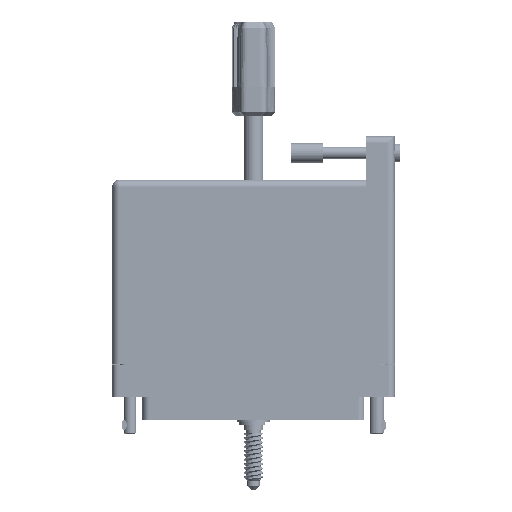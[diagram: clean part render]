
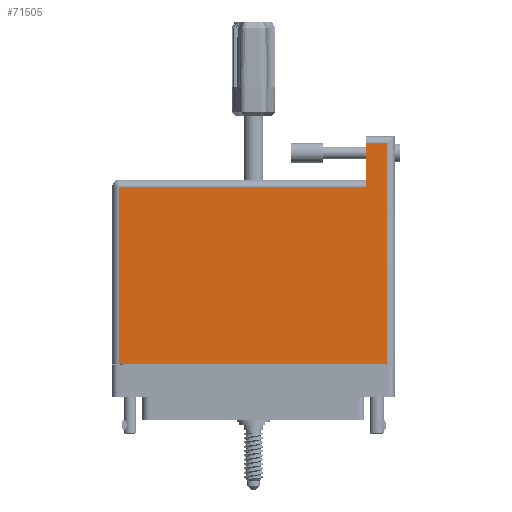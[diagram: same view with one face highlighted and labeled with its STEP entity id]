
A CAD part, front view. The second image highlights one B-rep face of the part: STEP entity #71505.
In plain terms, the highlighted face is planar.
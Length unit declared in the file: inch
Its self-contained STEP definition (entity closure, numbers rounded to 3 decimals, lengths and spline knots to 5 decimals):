
#1903 = ORIENTED_EDGE ( 'NONE', *, *, #75882, .T. ) ;
#1922 = VERTEX_POINT ( 'NONE', #93160 ) ;
#2564 = VERTEX_POINT ( 'NONE', #86191 ) ;
#4889 = VECTOR ( 'NONE', #37113, 39.37008 ) ;
#7090 = VECTOR ( 'NONE', #66469, 39.37008 ) ;
#7137 = CARTESIAN_POINT ( 'NONE',  ( 1.289, -0.1, 0.617 ) ) ;
#7687 = LINE ( 'NONE', #44389, #44986 ) ;
#10917 = EDGE_CURVE ( 'NONE', #56091, #29595, #30748, .T. ) ;
#13269 = ORIENTED_EDGE ( 'NONE', *, *, #47690, .T. ) ;
#14155 = AXIS2_PLACEMENT_3D ( 'NONE', #52039, #90207, #36883 ) ;
#15061 = CARTESIAN_POINT ( 'NONE',  ( -1.359, 2.025, 0.617 ) ) ;
#16395 = LINE ( 'NONE', #59484, #85983 ) ;
#24014 = DIRECTION ( 'NONE',  ( 0., -1., 0. ) ) ;
#25259 = ORIENTED_EDGE ( 'NONE', *, *, #70990, .T. ) ;
#27114 = DIRECTION ( 'NONE',  ( 1., 0., 0. ) ) ;
#29595 = VERTEX_POINT ( 'NONE', #50216 ) ;
#30748 = LINE ( 'NONE', #73796, #7090 ) ;
#36883 = DIRECTION ( 'NONE',  ( -1., 0., 0. ) ) ;
#37003 = DIRECTION ( 'NONE',  ( 0., -1., 0. ) ) ;
#37113 = DIRECTION ( 'NONE',  ( -1., 0., 0. ) ) ;
#41360 = CARTESIAN_POINT ( 'NONE',  ( -1.289, -0.1, 0.617 ) ) ;
#44389 = CARTESIAN_POINT ( 'NONE',  ( 1.289, 2.095, 0.617 ) ) ;
#44986 = VECTOR ( 'NONE', #67366, 39.37008 ) ;
#45047 = CARTESIAN_POINT ( 'NONE',  ( -1.289, -0.1, 0.617 ) ) ;
#47378 = VECTOR ( 'NONE', #27114, 39.37008 ) ;
#47690 = EDGE_CURVE ( 'NONE', #53337, #94446, #69347, .T. ) ;
#50216 = CARTESIAN_POINT ( 'NONE',  ( -1.289, 1.605, 0.617 ) ) ;
#52039 = CARTESIAN_POINT ( 'NONE',  ( -1.359, 1.675, 0.617 ) ) ;
#53337 = VERTEX_POINT ( 'NONE', #41360 ) ;
#55334 = EDGE_CURVE ( 'NONE', #94446, #1922, #7687, .T. ) ;
#55707 = EDGE_LOOP ( 'NONE', ( #65837, #84971, #13269, #86578, #1903, #25259 ) ) ;
#56091 = VERTEX_POINT ( 'NONE', #71416 ) ;
#59484 = CARTESIAN_POINT ( 'NONE',  ( 1.079, 2.095, 0.617 ) ) ;
#61032 = LINE ( 'NONE', #15061, #4889 ) ;
#65837 = ORIENTED_EDGE ( 'NONE', *, *, #10917, .T. ) ;
#66469 = DIRECTION ( 'NONE',  ( -1., 0., 0. ) ) ;
#67366 = DIRECTION ( 'NONE',  ( 0., 1., 0. ) ) ;
#67667 = PLANE ( 'NONE',  #14155 ) ;
#69347 = LINE ( 'NONE', #91891, #47378 ) ;
#70990 = EDGE_CURVE ( 'NONE', #2564, #56091, #16395, .T. ) ;
#71416 = CARTESIAN_POINT ( 'NONE',  ( 1.079, 1.605, 0.617 ) ) ;
#71505 = ADVANCED_FACE ( 'NONE', ( #90671 ), #67667, .F. ) ;
#73796 = CARTESIAN_POINT ( 'NONE',  ( -1.359, 1.605, 0.617 ) ) ;
#75882 = EDGE_CURVE ( 'NONE', #1922, #2564, #61032, .T. ) ;
#84971 = ORIENTED_EDGE ( 'NONE', *, *, #85835, .T. ) ;
#85835 = EDGE_CURVE ( 'NONE', #29595, #53337, #91032, .T. ) ;
#85983 = VECTOR ( 'NONE', #37003, 39.37008 ) ;
#86191 = CARTESIAN_POINT ( 'NONE',  ( 1.079, 2.025, 0.617 ) ) ;
#86578 = ORIENTED_EDGE ( 'NONE', *, *, #55334, .T. ) ;
#90207 = DIRECTION ( 'NONE',  ( 0., 0., -1. ) ) ;
#90671 = FACE_OUTER_BOUND ( 'NONE', #55707, .T. ) ;
#91032 = LINE ( 'NONE', #45047, #95441 ) ;
#91891 = CARTESIAN_POINT ( 'NONE',  ( -1.359, -0.1, 0.617 ) ) ;
#93160 = CARTESIAN_POINT ( 'NONE',  ( 1.289, 2.025, 0.617 ) ) ;
#94446 = VERTEX_POINT ( 'NONE', #7137 ) ;
#95441 = VECTOR ( 'NONE', #24014, 39.37008 ) ;
